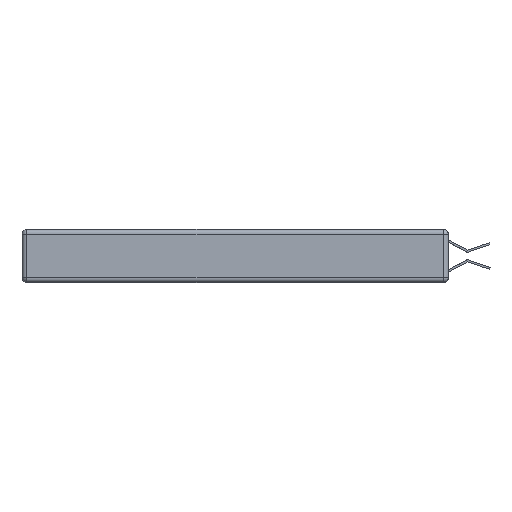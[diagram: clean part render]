
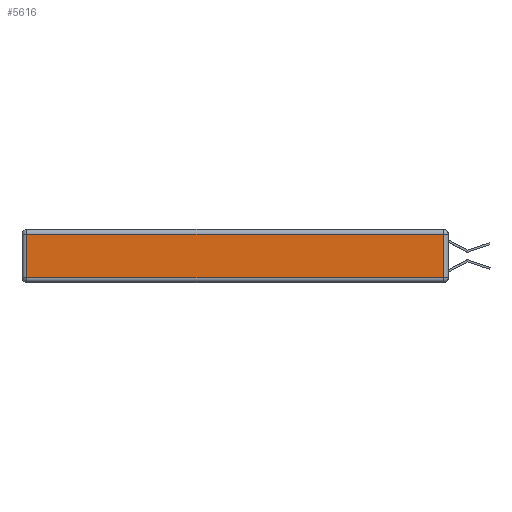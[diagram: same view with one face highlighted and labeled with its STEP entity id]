
A CAD part, left-side view. The second image highlights one B-rep face of the part: STEP entity #5616.
In plain terms, the highlighted planar face has unit normal (-1, 0, 0).
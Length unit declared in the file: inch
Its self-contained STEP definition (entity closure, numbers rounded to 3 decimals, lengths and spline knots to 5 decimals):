
#44 = DIRECTION ( 'NONE',  ( -1., 0., 0. ) ) ;
#217 = VECTOR ( 'NONE', #6572, 39.37008 ) ;
#767 = DIRECTION ( 'NONE',  ( 0., 1., 0. ) ) ;
#1087 = CARTESIAN_POINT ( 'NONE',  ( 0., 0., -0.313 ) ) ;
#1475 = DIRECTION ( 'NONE',  ( 0., 0., 1. ) ) ;
#1753 = VECTOR ( 'NONE', #5750, 39.37008 ) ;
#3329 = ORIENTED_EDGE ( 'NONE', *, *, #8135, .T. ) ;
#3870 = LINE ( 'NONE', #6342, #11208 ) ;
#4062 = CARTESIAN_POINT ( 'NONE',  ( 0., 0., -0.343 ) ) ;
#5155 = CARTESIAN_POINT ( 'NONE',  ( 0., 2.72, -0.03 ) ) ;
#5448 = VERTEX_POINT ( 'NONE', #5155 ) ;
#5616 = ADVANCED_FACE ( 'NONE', ( #10860 ), #14566, .T. ) ;
#5706 = CARTESIAN_POINT ( 'NONE',  ( 0., 0.03, -0.313 ) ) ;
#5750 = DIRECTION ( 'NONE',  ( 0., 0., -1. ) ) ;
#6144 = VECTOR ( 'NONE', #767, 39.37008 ) ;
#6342 = CARTESIAN_POINT ( 'NONE',  ( 0., 0.03, -0.343 ) ) ;
#6572 = DIRECTION ( 'NONE',  ( 0., -1., 0. ) ) ;
#7033 = VERTEX_POINT ( 'NONE', #5706 ) ;
#7648 = CARTESIAN_POINT ( 'NONE',  ( 0., 0.03, -0.03 ) ) ;
#8135 = EDGE_CURVE ( 'NONE', #5448, #12130, #11997, .T. ) ;
#8342 = ORIENTED_EDGE ( 'NONE', *, *, #15932, .T. ) ;
#8594 = CARTESIAN_POINT ( 'NONE',  ( 0., 2.75, -0.03 ) ) ;
#10326 = CARTESIAN_POINT ( 'NONE',  ( 0., 2.72, -0.313 ) ) ;
#10860 = FACE_OUTER_BOUND ( 'NONE', #11871, .T. ) ;
#11208 = VECTOR ( 'NONE', #12011, 39.37008 ) ;
#11871 = EDGE_LOOP ( 'NONE', ( #13032, #8342, #14113, #3329 ) ) ;
#11947 = VERTEX_POINT ( 'NONE', #7648 ) ;
#11997 = LINE ( 'NONE', #13735, #1753 ) ;
#12011 = DIRECTION ( 'NONE',  ( 0., 0., 1. ) ) ;
#12130 = VERTEX_POINT ( 'NONE', #10326 ) ;
#12917 = AXIS2_PLACEMENT_3D ( 'NONE', #4062, #44, #1475 ) ;
#13032 = ORIENTED_EDGE ( 'NONE', *, *, #13767, .T. ) ;
#13114 = LINE ( 'NONE', #8594, #6144 ) ;
#13735 = CARTESIAN_POINT ( 'NONE',  ( 0., 2.72, -0.343 ) ) ;
#13767 = EDGE_CURVE ( 'NONE', #12130, #7033, #15561, .T. ) ;
#14113 = ORIENTED_EDGE ( 'NONE', *, *, #14254, .T. ) ;
#14254 = EDGE_CURVE ( 'NONE', #11947, #5448, #13114, .T. ) ;
#14566 = PLANE ( 'NONE',  #12917 ) ;
#15561 = LINE ( 'NONE', #1087, #217 ) ;
#15932 = EDGE_CURVE ( 'NONE', #7033, #11947, #3870, .T. ) ;
